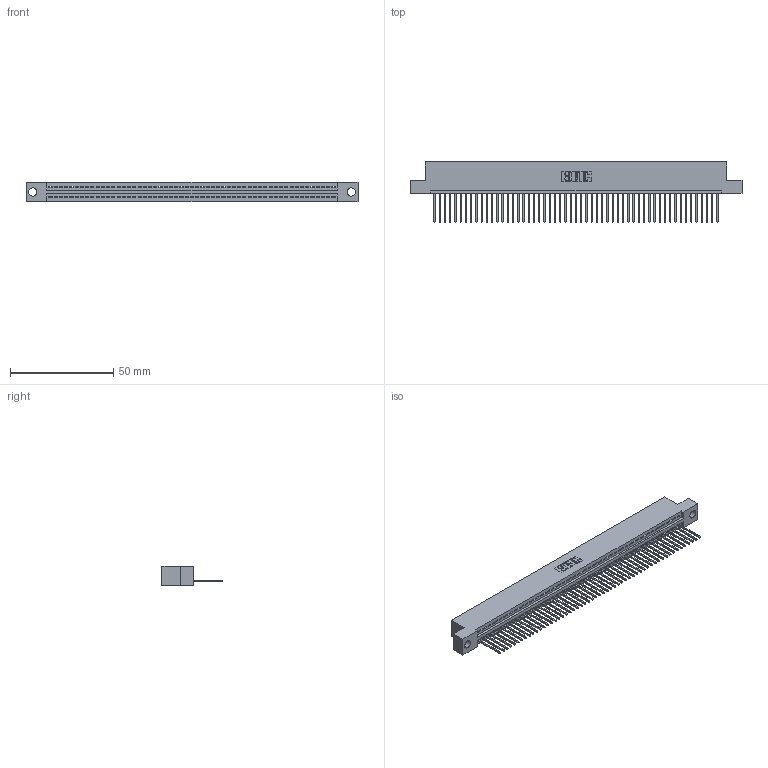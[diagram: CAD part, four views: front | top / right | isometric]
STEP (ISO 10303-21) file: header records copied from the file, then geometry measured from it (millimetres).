
FILE_DESCRIPTION (( 'STEP AP203' ), '1' );
FILE_NAME ('345-055-540-104.STEP', '2021-05-28T15:34:46', ( '' ), ( '' ), 'SwSTEP 2.0', 'SolidWorks 2020', '' );
FILE_SCHEMA (( 'CONFIG_CONTROL_DESIGN' ));
Length unit declared in the file: inch
Products named in the file (3): 345-292-001_345-293-140; 345 Part_Flush Mounting Lugs - 0.156 Dia-TI; 345-055-540-104
Assembly tree (56 placements, depth 2):
  345-055-540-104
    345 Part_Flush Mounting Lugs - 0.156 Dia-TI
    345-292-001_345-293-140  x55
Bounding box: 160.91 x 29.13 x 9.4 mm (x, y, z)
Volume: 15358.3 mm3; surface area: 20964.9 mm2
Topology: 56 solids, 56 shells, 3330 faces, 10057 edges, 6630 vertices
Faces by surface type: plane 2294, cylinder 1036
Entity records: 40081 total; most frequent: CARTESIAN_POINT 6951, ORIENTED_EDGE 6938, DIRECTION 6051, EDGE_CURVE 3469, LINE 3117, VECTOR 3117, VERTEX_POINT 2310, AXIS2_PLACEMENT_3D 1467
